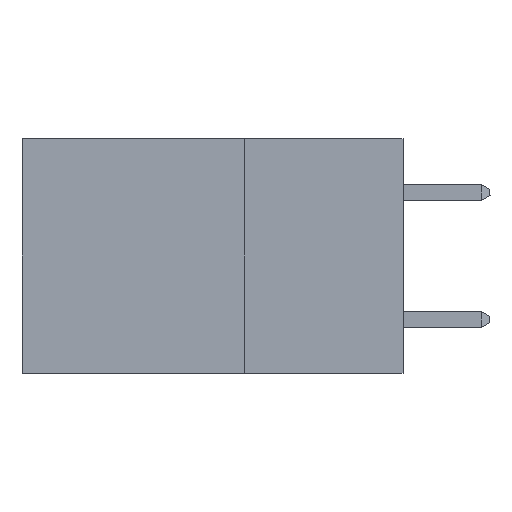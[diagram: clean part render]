
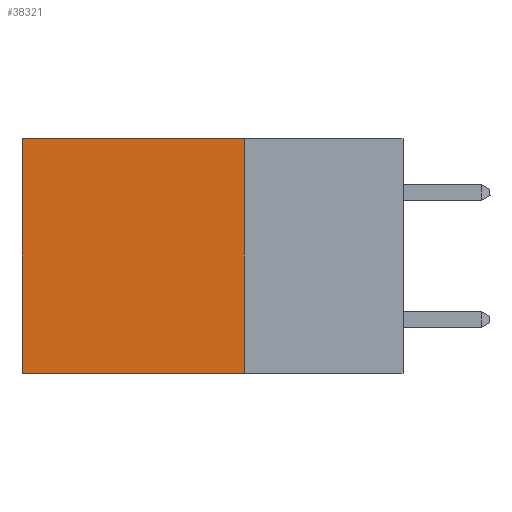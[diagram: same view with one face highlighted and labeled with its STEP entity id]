
A CAD part, left-side view. The second image highlights one B-rep face of the part: STEP entity #38321.
In plain terms, the highlighted planar face has unit normal (-1, 0, 0).
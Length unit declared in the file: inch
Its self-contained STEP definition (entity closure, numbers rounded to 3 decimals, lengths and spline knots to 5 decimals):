
#1177 = CARTESIAN_POINT ( 'NONE',  ( 0.2875, 0.25, -0.37 ) ) ;
#1493 = CARTESIAN_POINT ( 'NONE',  ( 0.2875, 0.25, 0. ) ) ;
#1575 = ORIENTED_EDGE ( 'NONE', *, *, #13191, .F. ) ;
#1713 = DIRECTION ( 'NONE',  ( 1., 0., 0. ) ) ;
#3641 = VECTOR ( 'NONE', #28225, 39.37008 ) ;
#3801 = VECTOR ( 'NONE', #36869, 39.37008 ) ;
#4164 = LINE ( 'NONE', #1177, #3641 ) ;
#4858 = LINE ( 'NONE', #1493, #37336 ) ;
#6648 = CARTESIAN_POINT ( 'NONE',  ( 0.2875, 0.6, 0. ) ) ;
#7618 = CARTESIAN_POINT ( 'NONE',  ( 0.2875, 0.25, -0.37 ) ) ;
#8194 = EDGE_CURVE ( 'NONE', #34119, #28404, #37265, .T. ) ;
#10137 = LINE ( 'NONE', #19891, #16368 ) ;
#10513 = EDGE_LOOP ( 'NONE', ( #17125, #1575, #17264, #35371 ) ) ;
#10676 = PLANE ( 'NONE',  #23556 ) ;
#12148 = CARTESIAN_POINT ( 'NONE',  ( 0.2875, 0.25, 0. ) ) ;
#13191 = EDGE_CURVE ( 'NONE', #23659, #28404, #4164, .T. ) ;
#14398 = DIRECTION ( 'NONE',  ( 0., 1., 0. ) ) ;
#15791 = VERTEX_POINT ( 'NONE', #12148 ) ;
#16368 = VECTOR ( 'NONE', #34591, 39.37008 ) ;
#17125 = ORIENTED_EDGE ( 'NONE', *, *, #8194, .T. ) ;
#17264 = ORIENTED_EDGE ( 'NONE', *, *, #35059, .F. ) ;
#19631 = FACE_OUTER_BOUND ( 'NONE', #10513, .T. ) ;
#19891 = CARTESIAN_POINT ( 'NONE',  ( 0.2875, 0.25, 0. ) ) ;
#19979 = CARTESIAN_POINT ( 'NONE',  ( 0.2875, 0.6, 0. ) ) ;
#23556 = AXIS2_PLACEMENT_3D ( 'NONE', #34927, #1713, #25983 ) ;
#23659 = VERTEX_POINT ( 'NONE', #7618 ) ;
#25983 = DIRECTION ( 'NONE',  ( 0., 0., -1. ) ) ;
#28225 = DIRECTION ( 'NONE',  ( 0., 1., 0. ) ) ;
#28404 = VERTEX_POINT ( 'NONE', #36011 ) ;
#34119 = VERTEX_POINT ( 'NONE', #19979 ) ;
#34591 = DIRECTION ( 'NONE',  ( 0., 0., -1. ) ) ;
#34927 = CARTESIAN_POINT ( 'NONE',  ( 0.2875, 0.25, 0. ) ) ;
#35059 = EDGE_CURVE ( 'NONE', #15791, #23659, #10137, .T. ) ;
#35371 = ORIENTED_EDGE ( 'NONE', *, *, #35416, .T. ) ;
#35416 = EDGE_CURVE ( 'NONE', #15791, #34119, #4858, .T. ) ;
#36011 = CARTESIAN_POINT ( 'NONE',  ( 0.2875, 0.6, -0.37 ) ) ;
#36869 = DIRECTION ( 'NONE',  ( 0., 0., -1. ) ) ;
#37265 = LINE ( 'NONE', #6648, #3801 ) ;
#37336 = VECTOR ( 'NONE', #14398, 39.37008 ) ;
#38321 = ADVANCED_FACE ( 'NONE', ( #19631 ), #10676, .F. ) ;
